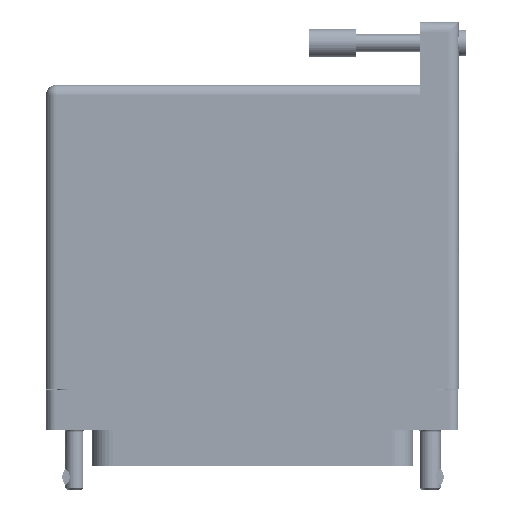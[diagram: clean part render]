
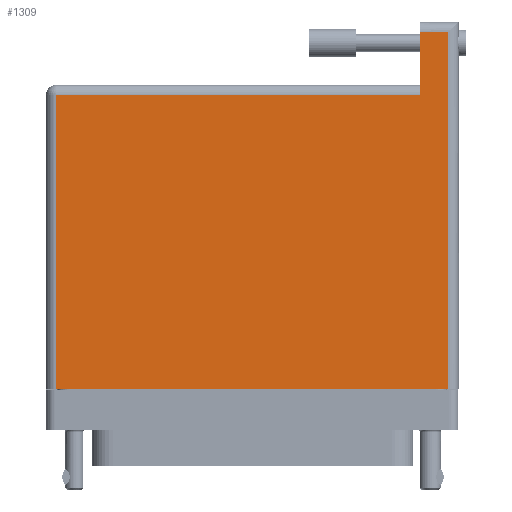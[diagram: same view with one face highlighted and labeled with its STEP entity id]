
A CAD part, front view. The second image highlights one B-rep face of the part: STEP entity #1309.
In plain terms, the highlighted face is planar.
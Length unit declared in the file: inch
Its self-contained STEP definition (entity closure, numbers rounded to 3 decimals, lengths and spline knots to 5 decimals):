
#341 = VERTEX_POINT ( 'NONE', #96604 ) ;
#571 = DIRECTION ( 'NONE',  ( 0., 1., 0. ) ) ;
#846 = EDGE_LOOP ( 'NONE', ( #102168, #55430, #27065, #80810, #64978, #46082 ) ) ;
#1309 = ADVANCED_FACE ( 'NONE', ( #12374 ), #6089, .F. ) ;
#6089 = PLANE ( 'NONE',  #75454 ) ;
#8356 = LINE ( 'NONE', #71847, #23686 ) ;
#9665 = EDGE_CURVE ( 'NONE', #87805, #42535, #85636, .T. ) ;
#10933 = VECTOR ( 'NONE', #95894, 39.37008 ) ;
#12374 = FACE_OUTER_BOUND ( 'NONE', #846, .T. ) ;
#13796 = CARTESIAN_POINT ( 'NONE',  ( -1.3075, 1.86, 0.765 ) ) ;
#14350 = DIRECTION ( 'NONE',  ( -1., 0., 0. ) ) ;
#14760 = CARTESIAN_POINT ( 'NONE',  ( -1.3775, 1.86, 0.765 ) ) ;
#22218 = VERTEX_POINT ( 'NONE', #32246 ) ;
#23686 = VECTOR ( 'NONE', #571, 39.37008 ) ;
#27065 = ORIENTED_EDGE ( 'NONE', *, *, #77630, .T. ) ;
#27851 = VECTOR ( 'NONE', #46965, 39.37008 ) ;
#32246 = CARTESIAN_POINT ( 'NONE',  ( 1.1215, 1.86, 0.765 ) ) ;
#32379 = LINE ( 'NONE', #62063, #27851 ) ;
#33393 = LINE ( 'NONE', #63620, #10933 ) ;
#37450 = VECTOR ( 'NONE', #45455, 39.37008 ) ;
#38157 = LINE ( 'NONE', #14760, #37450 ) ;
#38256 = CARTESIAN_POINT ( 'NONE',  ( -1.3775, 2.28, 0.765 ) ) ;
#41475 = EDGE_CURVE ( 'NONE', #42535, #22218, #33393, .T. ) ;
#42535 = VERTEX_POINT ( 'NONE', #83971 ) ;
#44118 = DIRECTION ( 'NONE',  ( 0., 0., -1. ) ) ;
#45309 = EDGE_CURVE ( 'NONE', #90530, #87805, #8356, .T. ) ;
#45455 = DIRECTION ( 'NONE',  ( -1., 0., 0. ) ) ;
#46082 = ORIENTED_EDGE ( 'NONE', *, *, #9665, .T. ) ;
#46965 = DIRECTION ( 'NONE',  ( 0., -1., 0. ) ) ;
#55430 = ORIENTED_EDGE ( 'NONE', *, *, #92215, .T. ) ;
#62063 = CARTESIAN_POINT ( 'NONE',  ( -1.3075, -0.1, 0.765 ) ) ;
#63620 = CARTESIAN_POINT ( 'NONE',  ( 1.1215, 2.35, 0.765 ) ) ;
#64978 = ORIENTED_EDGE ( 'NONE', *, *, #45309, .T. ) ;
#66819 = LINE ( 'NONE', #75126, #78036 ) ;
#71117 = CARTESIAN_POINT ( 'NONE',  ( 1.3075, -0.1, 0.765 ) ) ;
#71847 = CARTESIAN_POINT ( 'NONE',  ( 1.3075, 2.35, 0.765 ) ) ;
#75126 = CARTESIAN_POINT ( 'NONE',  ( -1.3775, -0.1, 0.765 ) ) ;
#75320 = CARTESIAN_POINT ( 'NONE',  ( -1.3775, 1.93, 0.765 ) ) ;
#75454 = AXIS2_PLACEMENT_3D ( 'NONE', #75320, #44118, #84700 ) ;
#77630 = EDGE_CURVE ( 'NONE', #85318, #341, #32379, .T. ) ;
#78036 = VECTOR ( 'NONE', #97581, 39.37008 ) ;
#80142 = EDGE_CURVE ( 'NONE', #341, #90530, #66819, .T. ) ;
#80810 = ORIENTED_EDGE ( 'NONE', *, *, #80142, .T. ) ;
#83971 = CARTESIAN_POINT ( 'NONE',  ( 1.1215, 2.28, 0.765 ) ) ;
#84700 = DIRECTION ( 'NONE',  ( -1., 0., 0. ) ) ;
#85318 = VERTEX_POINT ( 'NONE', #13796 ) ;
#85636 = LINE ( 'NONE', #38256, #97430 ) ;
#87805 = VERTEX_POINT ( 'NONE', #96182 ) ;
#90530 = VERTEX_POINT ( 'NONE', #71117 ) ;
#92215 = EDGE_CURVE ( 'NONE', #22218, #85318, #38157, .T. ) ;
#95894 = DIRECTION ( 'NONE',  ( 0., -1., 0. ) ) ;
#96182 = CARTESIAN_POINT ( 'NONE',  ( 1.3075, 2.28, 0.765 ) ) ;
#96604 = CARTESIAN_POINT ( 'NONE',  ( -1.3075, -0.1, 0.765 ) ) ;
#97430 = VECTOR ( 'NONE', #14350, 39.37008 ) ;
#97581 = DIRECTION ( 'NONE',  ( 1., 0., 0. ) ) ;
#102168 = ORIENTED_EDGE ( 'NONE', *, *, #41475, .T. ) ;
